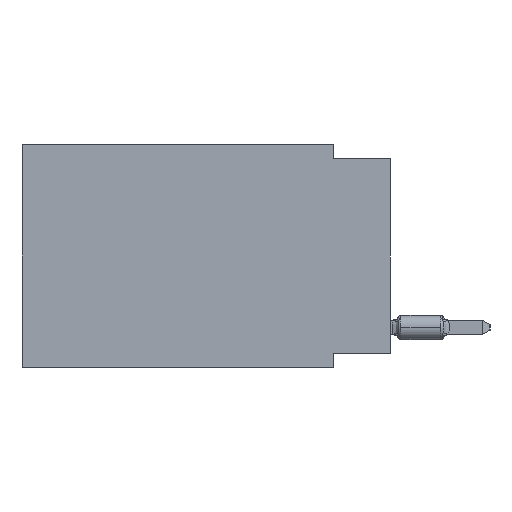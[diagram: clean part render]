
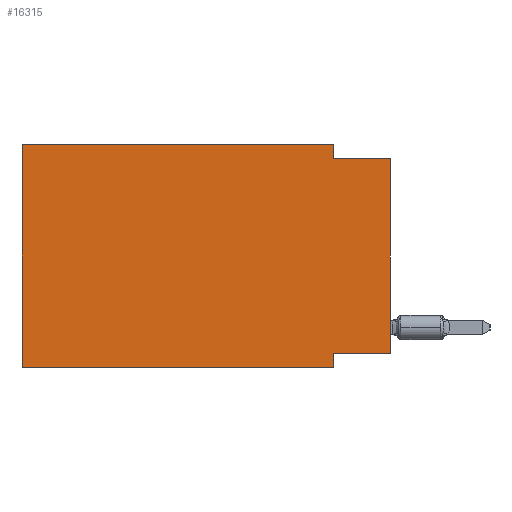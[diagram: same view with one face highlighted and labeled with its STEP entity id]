
A CAD part, left-side view. The second image highlights one B-rep face of the part: STEP entity #16315.
In plain terms, the highlighted planar face has unit normal (-1, 0, 0).
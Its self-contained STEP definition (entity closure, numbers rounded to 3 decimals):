
#110 = VECTOR ( 'NONE', #8013, 1000. ) ;
#629 = CARTESIAN_POINT ( 'NONE',  ( 0., 2.54, -0.635 ) ) ;
#1156 = VERTEX_POINT ( 'NONE', #21531 ) ;
#1505 = DIRECTION ( 'NONE',  ( 0., 0., -1. ) ) ;
#2541 = ORIENTED_EDGE ( 'NONE', *, *, #28009, .T. ) ;
#4060 = EDGE_CURVE ( 'NONE', #21351, #1156, #29561, .T. ) ;
#4389 = ORIENTED_EDGE ( 'NONE', *, *, #42584, .F. ) ;
#4762 = VERTEX_POINT ( 'NONE', #22387 ) ;
#5034 = CARTESIAN_POINT ( 'NONE',  ( 0., 2.54, -9.906 ) ) ;
#5632 = VERTEX_POINT ( 'NONE', #16342 ) ;
#6125 = CARTESIAN_POINT ( 'NONE',  ( 0., 16.383, 0. ) ) ;
#6255 = DIRECTION ( 'NONE',  ( 0., 1., 0. ) ) ;
#7857 = DIRECTION ( 'NONE',  ( 0., -1., 0. ) ) ;
#8013 = DIRECTION ( 'NONE',  ( 0., -1., 0. ) ) ;
#8836 = ORIENTED_EDGE ( 'NONE', *, *, #30774, .F. ) ;
#9513 = CARTESIAN_POINT ( 'NONE',  ( 0., 0., -9.271 ) ) ;
#9519 = VECTOR ( 'NONE', #6255, 1000. ) ;
#11020 = LINE ( 'NONE', #31232, #18662 ) ;
#11963 = VECTOR ( 'NONE', #20869, 1000. ) ;
#12170 = CARTESIAN_POINT ( 'NONE',  ( 0., 2.54, -9.906 ) ) ;
#13055 = DIRECTION ( 'NONE',  ( 1., 0., 0. ) ) ;
#13469 = CARTESIAN_POINT ( 'NONE',  ( 0., 0., -9.271 ) ) ;
#13692 = CARTESIAN_POINT ( 'NONE',  ( 0., 16.383, -9.906 ) ) ;
#14087 = LINE ( 'NONE', #41229, #38422 ) ;
#15252 = EDGE_CURVE ( 'NONE', #5632, #41828, #14087, .T. ) ;
#16315 = ADVANCED_FACE ( 'NONE', ( #22626 ), #30017, .F. ) ;
#16342 = CARTESIAN_POINT ( 'NONE',  ( 0., 2.54, 0. ) ) ;
#16553 = EDGE_CURVE ( 'NONE', #21351, #42560, #18054, .T. ) ;
#16607 = CARTESIAN_POINT ( 'NONE',  ( 0., 0., -0.635 ) ) ;
#17809 = VERTEX_POINT ( 'NONE', #13469 ) ;
#18054 = LINE ( 'NONE', #37368, #11963 ) ;
#18662 = VECTOR ( 'NONE', #31657, 1000. ) ;
#20653 = LINE ( 'NONE', #34127, #25539 ) ;
#20869 = DIRECTION ( 'NONE',  ( 0., -1., 0. ) ) ;
#21351 = VERTEX_POINT ( 'NONE', #13692 ) ;
#21531 = CARTESIAN_POINT ( 'NONE',  ( 0., 16.383, 0. ) ) ;
#21752 = AXIS2_PLACEMENT_3D ( 'NONE', #6125, #13055, #42798 ) ;
#21863 = EDGE_CURVE ( 'NONE', #1156, #5632, #24520, .T. ) ;
#22387 = CARTESIAN_POINT ( 'NONE',  ( 0., 2.54, -9.271 ) ) ;
#22626 = FACE_OUTER_BOUND ( 'NONE', #24893, .T. ) ;
#23343 = ORIENTED_EDGE ( 'NONE', *, *, #24624, .F. ) ;
#24520 = LINE ( 'NONE', #37757, #110 ) ;
#24624 = EDGE_CURVE ( 'NONE', #17809, #4762, #26026, .T. ) ;
#24893 = EDGE_LOOP ( 'NONE', ( #2541, #4389, #27423, #36368, #29477, #30885, #8836, #23343 ) ) ;
#25539 = VECTOR ( 'NONE', #7857, 1000. ) ;
#26026 = LINE ( 'NONE', #9513, #9519 ) ;
#26302 = DIRECTION ( 'NONE',  ( 0., 0., 1. ) ) ;
#27287 = VERTEX_POINT ( 'NONE', #16607 ) ;
#27423 = ORIENTED_EDGE ( 'NONE', *, *, #15252, .F. ) ;
#28009 = EDGE_CURVE ( 'NONE', #17809, #27287, #11020, .T. ) ;
#28263 = DIRECTION ( 'NONE',  ( 0., 0., -1. ) ) ;
#29477 = ORIENTED_EDGE ( 'NONE', *, *, #4060, .F. ) ;
#29561 = LINE ( 'NONE', #36269, #42460 ) ;
#30017 = PLANE ( 'NONE',  #21752 ) ;
#30774 = EDGE_CURVE ( 'NONE', #4762, #42560, #41918, .T. ) ;
#30885 = ORIENTED_EDGE ( 'NONE', *, *, #16553, .T. ) ;
#31232 = CARTESIAN_POINT ( 'NONE',  ( 0., 0., 0. ) ) ;
#31657 = DIRECTION ( 'NONE',  ( 0., 0., 1. ) ) ;
#34127 = CARTESIAN_POINT ( 'NONE',  ( 0., 0., -0.635 ) ) ;
#36269 = CARTESIAN_POINT ( 'NONE',  ( 0., 16.383, 0. ) ) ;
#36368 = ORIENTED_EDGE ( 'NONE', *, *, #21863, .F. ) ;
#37368 = CARTESIAN_POINT ( 'NONE',  ( 0., 16.383, -9.906 ) ) ;
#37757 = CARTESIAN_POINT ( 'NONE',  ( 0., 16.383, 0. ) ) ;
#38422 = VECTOR ( 'NONE', #1505, 1000. ) ;
#38580 = VECTOR ( 'NONE', #28263, 1000. ) ;
#41229 = CARTESIAN_POINT ( 'NONE',  ( 0., 2.54, 0. ) ) ;
#41828 = VERTEX_POINT ( 'NONE', #629 ) ;
#41918 = LINE ( 'NONE', #12170, #38580 ) ;
#42460 = VECTOR ( 'NONE', #26302, 1000. ) ;
#42560 = VERTEX_POINT ( 'NONE', #5034 ) ;
#42584 = EDGE_CURVE ( 'NONE', #41828, #27287, #20653, .T. ) ;
#42798 = DIRECTION ( 'NONE',  ( 0., 0., -1. ) ) ;
